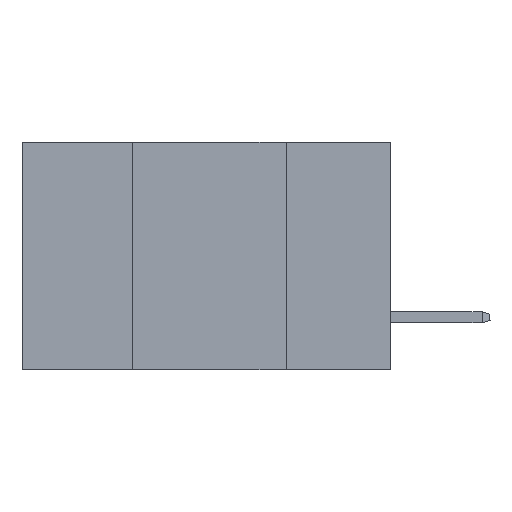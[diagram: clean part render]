
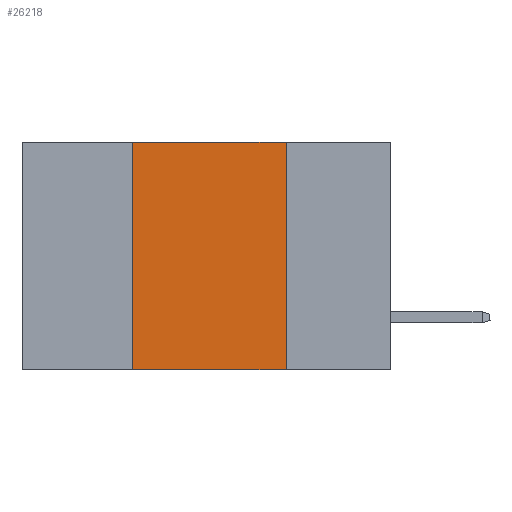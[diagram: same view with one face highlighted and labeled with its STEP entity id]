
A CAD part, left-side view. The second image highlights one B-rep face of the part: STEP entity #26218.
In plain terms, the highlighted planar face has unit normal (-1, 0, 0).
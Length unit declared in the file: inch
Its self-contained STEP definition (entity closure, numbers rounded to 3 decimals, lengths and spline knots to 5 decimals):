
#652 = VERTEX_POINT ( 'NONE', #672 ) ;
#672 = CARTESIAN_POINT ( 'NONE',  ( 0., 0.42, 0. ) ) ;
#858 = VERTEX_POINT ( 'NONE', #18425 ) ;
#2839 = CARTESIAN_POINT ( 'NONE',  ( 0., 0.6, -0.37 ) ) ;
#2927 = DIRECTION ( 'NONE',  ( 0., -1., 0. ) ) ;
#4502 = PLANE ( 'NONE',  #10924 ) ;
#4727 = VECTOR ( 'NONE', #21794, 39.37008 ) ;
#5206 = VERTEX_POINT ( 'NONE', #10316 ) ;
#5329 = LINE ( 'NONE', #13588, #11488 ) ;
#5761 = ORIENTED_EDGE ( 'NONE', *, *, #11023, .F. ) ;
#6969 = VERTEX_POINT ( 'NONE', #19622 ) ;
#8844 = ORIENTED_EDGE ( 'NONE', *, *, #11593, .F. ) ;
#9276 = LINE ( 'NONE', #2839, #10246 ) ;
#10246 = VECTOR ( 'NONE', #2927, 39.37008 ) ;
#10255 = LINE ( 'NONE', #19968, #4727 ) ;
#10316 = CARTESIAN_POINT ( 'NONE',  ( 0., 0.17, 0. ) ) ;
#10924 = AXIS2_PLACEMENT_3D ( 'NONE', #14999, #21378, #11002 ) ;
#11002 = DIRECTION ( 'NONE',  ( 0., 0., -1. ) ) ;
#11023 = EDGE_CURVE ( 'NONE', #6969, #652, #10255, .T. ) ;
#11488 = VECTOR ( 'NONE', #17955, 39.37008 ) ;
#11523 = EDGE_CURVE ( 'NONE', #5206, #858, #23503, .T. ) ;
#11593 = EDGE_CURVE ( 'NONE', #652, #5206, #5329, .T. ) ;
#13588 = CARTESIAN_POINT ( 'NONE',  ( 0., 0.6, 0. ) ) ;
#13728 = ORIENTED_EDGE ( 'NONE', *, *, #11523, .F. ) ;
#14999 = CARTESIAN_POINT ( 'NONE',  ( 0., 0.6, 0. ) ) ;
#15363 = EDGE_CURVE ( 'NONE', #6969, #858, #9276, .T. ) ;
#17646 = CARTESIAN_POINT ( 'NONE',  ( 0., 0.17, 0. ) ) ;
#17955 = DIRECTION ( 'NONE',  ( 0., -1., 0. ) ) ;
#18425 = CARTESIAN_POINT ( 'NONE',  ( 0., 0.17, -0.37 ) ) ;
#19622 = CARTESIAN_POINT ( 'NONE',  ( 0., 0.42, -0.37 ) ) ;
#19968 = CARTESIAN_POINT ( 'NONE',  ( 0., 0.42, 0. ) ) ;
#20281 = VECTOR ( 'NONE', #23803, 39.37008 ) ;
#21378 = DIRECTION ( 'NONE',  ( 1., 0., 0. ) ) ;
#21794 = DIRECTION ( 'NONE',  ( 0., 0., 1. ) ) ;
#22447 = FACE_OUTER_BOUND ( 'NONE', #23286, .T. ) ;
#22496 = ORIENTED_EDGE ( 'NONE', *, *, #15363, .T. ) ;
#23286 = EDGE_LOOP ( 'NONE', ( #13728, #8844, #5761, #22496 ) ) ;
#23503 = LINE ( 'NONE', #17646, #20281 ) ;
#23803 = DIRECTION ( 'NONE',  ( 0., 0., -1. ) ) ;
#26218 = ADVANCED_FACE ( 'NONE', ( #22447 ), #4502, .F. ) ;
